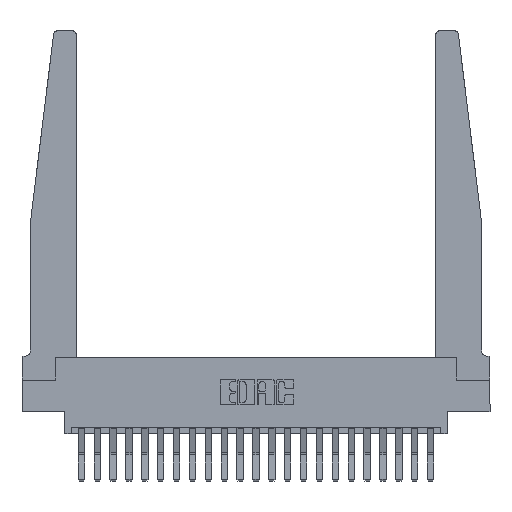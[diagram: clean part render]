
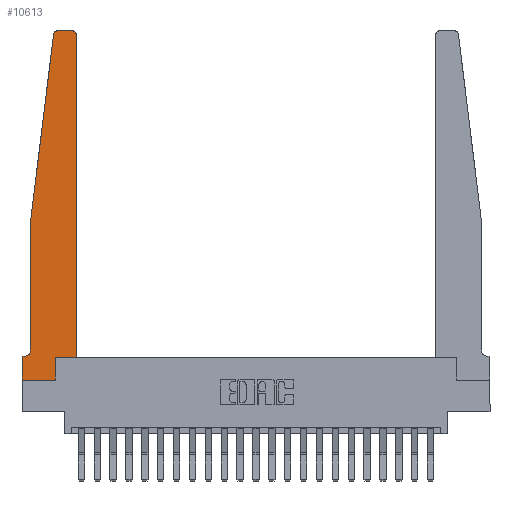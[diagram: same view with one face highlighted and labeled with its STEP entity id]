
A CAD part, top view. The second image highlights one B-rep face of the part: STEP entity #10613.
In plain terms, the highlighted planar face has unit normal (0, 0, 1).
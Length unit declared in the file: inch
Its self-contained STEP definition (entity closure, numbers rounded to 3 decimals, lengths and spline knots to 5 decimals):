
#98 = VECTOR ( 'NONE', #19293, 39.37008 ) ;
#107 = DIRECTION ( 'NONE',  ( 0., 0., -1. ) ) ;
#177 = LINE ( 'NONE', #8544, #8942 ) ;
#319 = EDGE_CURVE ( 'NONE', #8043, #1247, #21762, .T. ) ;
#573 = LINE ( 'NONE', #3911, #4700 ) ;
#652 = VECTOR ( 'NONE', #19723, 39.37008 ) ;
#1247 = VERTEX_POINT ( 'NONE', #10335 ) ;
#1387 = DIRECTION ( 'NONE',  ( -1., 0., 0. ) ) ;
#1626 = EDGE_CURVE ( 'NONE', #3090, #21759, #10347, .T. ) ;
#1829 = VERTEX_POINT ( 'NONE', #6618 ) ;
#2368 = EDGE_CURVE ( 'NONE', #14433, #5641, #177, .T. ) ;
#2614 = CARTESIAN_POINT ( 'NONE',  ( 0.425, 0.18, 0.37 ) ) ;
#2709 = CARTESIAN_POINT ( 'NONE',  ( 0.2605, 0., 0.37 ) ) ;
#2785 = LINE ( 'NONE', #19287, #20772 ) ;
#3090 = VERTEX_POINT ( 'NONE', #15386 ) ;
#3911 = CARTESIAN_POINT ( 'NONE',  ( 0., 0., 0.37 ) ) ;
#4269 = VERTEX_POINT ( 'NONE', #10519 ) ;
#4301 = EDGE_CURVE ( 'NONE', #4269, #8043, #5351, .T. ) ;
#4590 = ORIENTED_EDGE ( 'NONE', *, *, #15388, .T. ) ;
#4696 = FACE_OUTER_BOUND ( 'NONE', #8206, .T. ) ;
#4700 = VECTOR ( 'NONE', #12580, 39.37008 ) ;
#4747 = VECTOR ( 'NONE', #16073, 39.37008 ) ;
#5124 = CARTESIAN_POINT ( 'NONE',  ( 0.27653, 2.72, 0.37 ) ) ;
#5162 = CARTESIAN_POINT ( 'NONE',  ( 0.395, 2.72, 0.37 ) ) ;
#5309 = CARTESIAN_POINT ( 'NONE',  ( 0.015, 0.1875, 0.37 ) ) ;
#5342 = LINE ( 'NONE', #16206, #652 ) ;
#5351 = LINE ( 'NONE', #10592, #98 ) ;
#5641 = VERTEX_POINT ( 'NONE', #16392 ) ;
#5738 = VECTOR ( 'NONE', #13046, 39.37008 ) ;
#6163 = ORIENTED_EDGE ( 'NONE', *, *, #1626, .T. ) ;
#6575 = AXIS2_PLACEMENT_3D ( 'NONE', #17454, #19215, #8755 ) ;
#6618 = CARTESIAN_POINT ( 'NONE',  ( 0.395, 2.75, 0.37 ) ) ;
#6862 = LINE ( 'NONE', #20601, #11456 ) ;
#6871 = DIRECTION ( 'NONE',  ( 1., 0., 0. ) ) ;
#6914 = DIRECTION ( 'NONE',  ( 1., 0., 0. ) ) ;
#6951 = CARTESIAN_POINT ( 'NONE',  ( 0.27653, 2.75, 0.37 ) ) ;
#7101 = DIRECTION ( 'NONE',  ( 0., 1., 0. ) ) ;
#7219 = ORIENTED_EDGE ( 'NONE', *, *, #11859, .T. ) ;
#7433 = ORIENTED_EDGE ( 'NONE', *, *, #2368, .T. ) ;
#7633 = ORIENTED_EDGE ( 'NONE', *, *, #16085, .T. ) ;
#7775 = DIRECTION ( 'NONE',  ( 0., -1., 0. ) ) ;
#7929 = EDGE_CURVE ( 'NONE', #10198, #14433, #5342, .T. ) ;
#8043 = VERTEX_POINT ( 'NONE', #9585 ) ;
#8206 = EDGE_LOOP ( 'NONE', ( #20508, #4590, #15124, #11897, #18262, #16312, #7433, #14829, #9889, #6163, #7633, #7219 ) ) ;
#8544 = CARTESIAN_POINT ( 'NONE',  ( 0., 0., 0.37 ) ) ;
#8755 = DIRECTION ( 'NONE',  ( 1., 0., 0. ) ) ;
#8942 = VECTOR ( 'NONE', #17248, 39.37008 ) ;
#9233 = CARTESIAN_POINT ( 'NONE',  ( 0.065, 1.25, 0.37 ) ) ;
#9585 = CARTESIAN_POINT ( 'NONE',  ( 0.065, 1.25, 0.37 ) ) ;
#9889 = ORIENTED_EDGE ( 'NONE', *, *, #14493, .T. ) ;
#10198 = VERTEX_POINT ( 'NONE', #5309 ) ;
#10335 = CARTESIAN_POINT ( 'NONE',  ( 0.065, 0.2375, 0.37 ) ) ;
#10347 = LINE ( 'NONE', #2614, #5738 ) ;
#10507 = AXIS2_PLACEMENT_3D ( 'NONE', #10587, #107, #12339 ) ;
#10519 = CARTESIAN_POINT ( 'NONE',  ( 0.24675, 2.72367, 0.37 ) ) ;
#10587 = CARTESIAN_POINT ( 'NONE',  ( 0.015, 0.2375, 0.37 ) ) ;
#10592 = CARTESIAN_POINT ( 'NONE',  ( 0.065, 1.25, 0.37 ) ) ;
#10613 = ADVANCED_FACE ( 'NONE', ( #4696 ), #15694, .T. ) ;
#10719 = VERTEX_POINT ( 'NONE', #12401 ) ;
#11456 = VECTOR ( 'NONE', #1387, 39.37008 ) ;
#11859 = EDGE_CURVE ( 'NONE', #10719, #1829, #17716, .T. ) ;
#11897 = ORIENTED_EDGE ( 'NONE', *, *, #319, .T. ) ;
#12237 = AXIS2_PLACEMENT_3D ( 'NONE', #5162, #17339, #6914 ) ;
#12339 = DIRECTION ( 'NONE',  ( -1., 0., 0. ) ) ;
#12401 = CARTESIAN_POINT ( 'NONE',  ( 0.425, 2.72, 0.37 ) ) ;
#12509 = VERTEX_POINT ( 'NONE', #6951 ) ;
#12580 = DIRECTION ( 'NONE',  ( 1., 0., 0. ) ) ;
#13020 = EDGE_CURVE ( 'NONE', #1247, #10198, #22531, .T. ) ;
#13046 = DIRECTION ( 'NONE',  ( 1., 0., 0. ) ) ;
#14321 = CARTESIAN_POINT ( 'NONE',  ( 0., 0.1875, 0.37 ) ) ;
#14433 = VERTEX_POINT ( 'NONE', #14321 ) ;
#14493 = EDGE_CURVE ( 'NONE', #20998, #3090, #18658, .T. ) ;
#14829 = ORIENTED_EDGE ( 'NONE', *, *, #15542, .T. ) ;
#15124 = ORIENTED_EDGE ( 'NONE', *, *, #4301, .T. ) ;
#15386 = CARTESIAN_POINT ( 'NONE',  ( 0.2605, 0.18, 0.37 ) ) ;
#15388 = EDGE_CURVE ( 'NONE', #12509, #4269, #16680, .T. ) ;
#15542 = EDGE_CURVE ( 'NONE', #5641, #20998, #573, .T. ) ;
#15694 = PLANE ( 'NONE',  #6575 ) ;
#16073 = DIRECTION ( 'NONE',  ( 0., 1., 0. ) ) ;
#16085 = EDGE_CURVE ( 'NONE', #21759, #10719, #2785, .T. ) ;
#16206 = CARTESIAN_POINT ( 'NONE',  ( 0.065, 0.1875, 0.37 ) ) ;
#16312 = ORIENTED_EDGE ( 'NONE', *, *, #7929, .T. ) ;
#16392 = CARTESIAN_POINT ( 'NONE',  ( 0., 0., 0.37 ) ) ;
#16680 = CIRCLE ( 'NONE', #20478, 0.03 ) ;
#17154 = EDGE_CURVE ( 'NONE', #1829, #12509, #6862, .T. ) ;
#17248 = DIRECTION ( 'NONE',  ( 0., -1., 0. ) ) ;
#17303 = DIRECTION ( 'NONE',  ( 0., 0., 1. ) ) ;
#17339 = DIRECTION ( 'NONE',  ( 0., 0., 1. ) ) ;
#17454 = CARTESIAN_POINT ( 'NONE',  ( 0., 0.1875, 0.37 ) ) ;
#17716 = CIRCLE ( 'NONE', #12237, 0.03 ) ;
#17928 = CARTESIAN_POINT ( 'NONE',  ( 0.2605, 0.18, 0.37 ) ) ;
#18262 = ORIENTED_EDGE ( 'NONE', *, *, #13020, .T. ) ;
#18658 = LINE ( 'NONE', #17928, #4747 ) ;
#19215 = DIRECTION ( 'NONE',  ( 0., 0., 1. ) ) ;
#19287 = CARTESIAN_POINT ( 'NONE',  ( 0.425, 0.18, 0.37 ) ) ;
#19293 = DIRECTION ( 'NONE',  ( -0.122, -0.992, 0. ) ) ;
#19723 = DIRECTION ( 'NONE',  ( -1., 0., 0. ) ) ;
#20478 = AXIS2_PLACEMENT_3D ( 'NONE', #5124, #17303, #6871 ) ;
#20508 = ORIENTED_EDGE ( 'NONE', *, *, #17154, .T. ) ;
#20601 = CARTESIAN_POINT ( 'NONE',  ( 0.25, 2.75, 0.37 ) ) ;
#20772 = VECTOR ( 'NONE', #7101, 39.37008 ) ;
#20998 = VERTEX_POINT ( 'NONE', #2709 ) ;
#21097 = CARTESIAN_POINT ( 'NONE',  ( 0.425, 0.18, 0.37 ) ) ;
#21225 = VECTOR ( 'NONE', #7775, 39.37008 ) ;
#21759 = VERTEX_POINT ( 'NONE', #21097 ) ;
#21762 = LINE ( 'NONE', #9233, #21225 ) ;
#22531 = CIRCLE ( 'NONE', #10507, 0.05 ) ;
